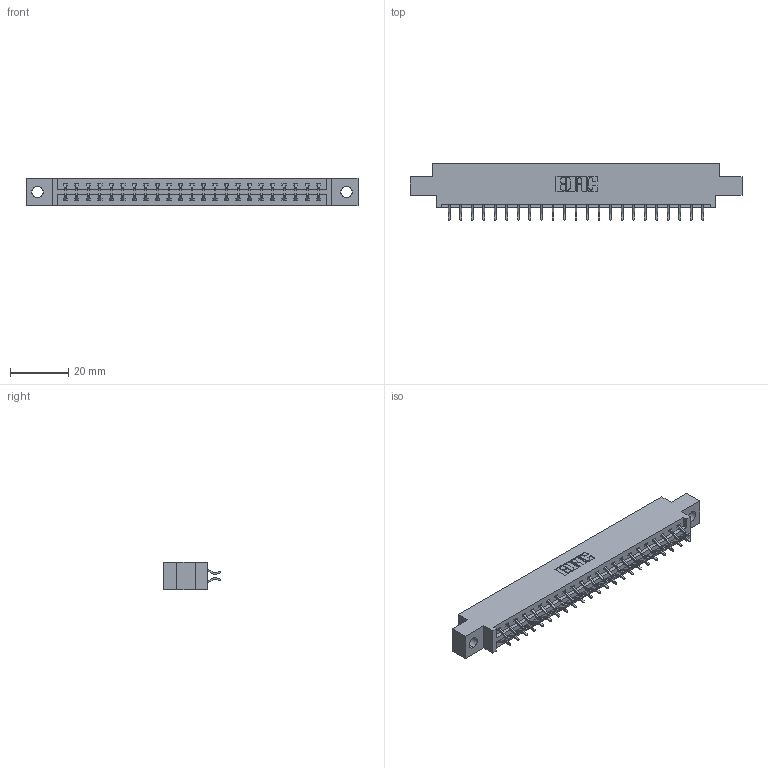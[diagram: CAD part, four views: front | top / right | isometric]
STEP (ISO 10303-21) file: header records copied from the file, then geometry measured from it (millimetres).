
FILE_DESCRIPTION (( 'STEP AP203' ), '1' );
FILE_NAME ('337-046-556-804.STEP', '2018-08-09T08:23:41', ( '' ), ( '' ), 'SwSTEP 2.0', 'SolidWorks 2016', '' );
FILE_SCHEMA (( 'CONFIG_CONTROL_DESIGN' ));
Length unit declared in the file: inch
Products named in the file (3): 337 Part_0.170 Offset - 0.156 Dia-TH; 345-292-001_556 Tail; 337-046-556-804
Assembly tree (47 placements, depth 2):
  337-046-556-804
    337 Part_0.170 Offset - 0.156 Dia-TH
    345-292-001_556 Tail  x46
Bounding box: 114.15 x 19.57 x 9.4 mm (x, y, z)
Volume: 11569.7 mm3; surface area: 12751.7 mm2
Topology: 47 solids, 47 shells, 2878 faces, 8557 edges, 5642 vertices
Faces by surface type: plane 2006, cylinder 872
Entity records: 20645 total; most frequent: CARTESIAN_POINT 3510, ORIENTED_EDGE 3434, DIRECTION 3009, EDGE_CURVE 1717, LINE 1581, VECTOR 1581, VERTEX_POINT 1142, AXIS2_PLACEMENT_3D 714
